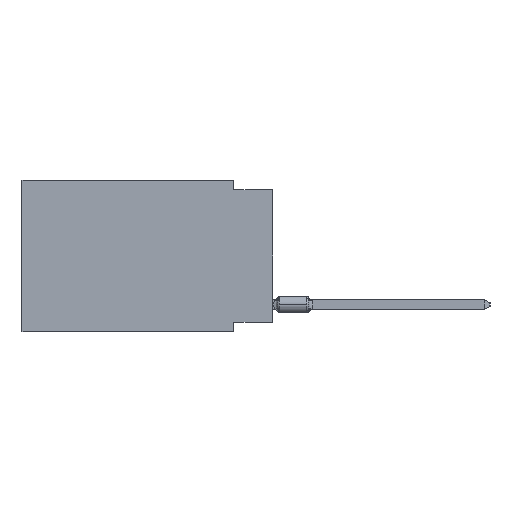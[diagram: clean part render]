
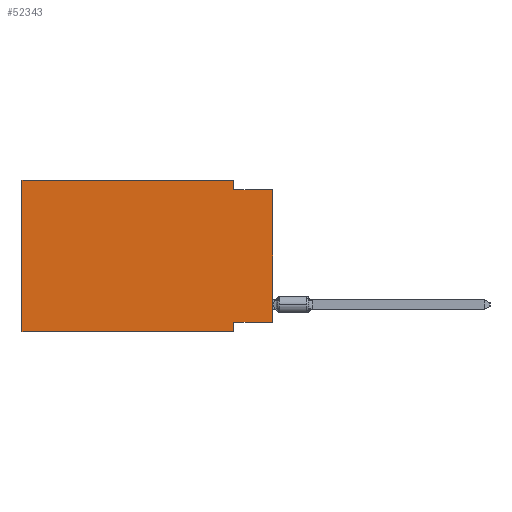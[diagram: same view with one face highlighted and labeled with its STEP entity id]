
A CAD part, left-side view. The second image highlights one B-rep face of the part: STEP entity #52343.
In plain terms, the highlighted planar face has unit normal (-1, 0, 0).
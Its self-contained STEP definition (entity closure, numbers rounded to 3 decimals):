
#439 = ORIENTED_EDGE ( 'NONE', *, *, #15975, .F. ) ;
#594 = DIRECTION ( 'NONE',  ( 0., -1., 0. ) ) ;
#1519 = DIRECTION ( 'NONE',  ( 1., 0., 0. ) ) ;
#2572 = EDGE_CURVE ( 'NONE', #44456, #15717, #60464, .T. ) ;
#2872 = DIRECTION ( 'NONE',  ( 0., 0., 1. ) ) ;
#3669 = CARTESIAN_POINT ( 'NONE',  ( 0., 16.383, 0. ) ) ;
#4310 = ORIENTED_EDGE ( 'NONE', *, *, #54827, .F. ) ;
#5152 = EDGE_CURVE ( 'NONE', #33757, #67316, #58648, .T. ) ;
#8845 = DIRECTION ( 'NONE',  ( 0., -1., 0. ) ) ;
#10815 = VECTOR ( 'NONE', #2872, 1000. ) ;
#11111 = CARTESIAN_POINT ( 'NONE',  ( 0., 2.54, -9.906 ) ) ;
#11464 = CARTESIAN_POINT ( 'NONE',  ( 0., 2.54, 0. ) ) ;
#12512 = VECTOR ( 'NONE', #8845, 1000. ) ;
#12862 = CARTESIAN_POINT ( 'NONE',  ( 0., 16.383, 0. ) ) ;
#13574 = DIRECTION ( 'NONE',  ( 0., -1., 0. ) ) ;
#13678 = LINE ( 'NONE', #3669, #12512 ) ;
#14468 = CARTESIAN_POINT ( 'NONE',  ( 0., 0., 0. ) ) ;
#15052 = CARTESIAN_POINT ( 'NONE',  ( 0., 2.54, -9.906 ) ) ;
#15717 = VERTEX_POINT ( 'NONE', #11111 ) ;
#15845 = CARTESIAN_POINT ( 'NONE',  ( 0., 0., -9.271 ) ) ;
#15975 = EDGE_CURVE ( 'NONE', #67316, #20374, #13678, .T. ) ;
#16639 = EDGE_CURVE ( 'NONE', #33757, #15717, #19100, .T. ) ;
#17919 = VECTOR ( 'NONE', #594, 1000. ) ;
#18137 = PLANE ( 'NONE',  #50820 ) ;
#19100 = LINE ( 'NONE', #41634, #67995 ) ;
#19553 = CARTESIAN_POINT ( 'NONE',  ( 0., 0., -0.635 ) ) ;
#19812 = DIRECTION ( 'NONE',  ( 0., 1., 0. ) ) ;
#20374 = VERTEX_POINT ( 'NONE', #34454 ) ;
#20508 = VERTEX_POINT ( 'NONE', #42528 ) ;
#24146 = ORIENTED_EDGE ( 'NONE', *, *, #67704, .F. ) ;
#27179 = LINE ( 'NONE', #29018, #17919 ) ;
#29018 = CARTESIAN_POINT ( 'NONE',  ( 0., 0., -0.635 ) ) ;
#30363 = VERTEX_POINT ( 'NONE', #19553 ) ;
#31337 = EDGE_CURVE ( 'NONE', #20374, #20508, #46146, .T. ) ;
#32254 = VECTOR ( 'NONE', #19812, 1000. ) ;
#33107 = DIRECTION ( 'NONE',  ( 0., 0., -1. ) ) ;
#33757 = VERTEX_POINT ( 'NONE', #69643 ) ;
#34454 = CARTESIAN_POINT ( 'NONE',  ( 0., 2.54, 0. ) ) ;
#36993 = DIRECTION ( 'NONE',  ( 0., 0., 1. ) ) ;
#38234 = ORIENTED_EDGE ( 'NONE', *, *, #31337, .F. ) ;
#41272 = LINE ( 'NONE', #52713, #32254 ) ;
#41634 = CARTESIAN_POINT ( 'NONE',  ( 0., 16.383, -9.906 ) ) ;
#42528 = CARTESIAN_POINT ( 'NONE',  ( 0., 2.54, -0.635 ) ) ;
#43493 = VECTOR ( 'NONE', #33107, 1000. ) ;
#44456 = VERTEX_POINT ( 'NONE', #46496 ) ;
#44555 = EDGE_LOOP ( 'NONE', ( #44778, #24146, #38234, #439, #54751, #67600, #47407, #4310 ) ) ;
#44778 = ORIENTED_EDGE ( 'NONE', *, *, #63929, .T. ) ;
#45044 = DIRECTION ( 'NONE',  ( 0., 0., -1. ) ) ;
#45253 = VECTOR ( 'NONE', #45044, 1000. ) ;
#45731 = CARTESIAN_POINT ( 'NONE',  ( 0., 16.383, 0. ) ) ;
#46146 = LINE ( 'NONE', #11464, #45253 ) ;
#46496 = CARTESIAN_POINT ( 'NONE',  ( 0., 2.54, -9.271 ) ) ;
#47407 = ORIENTED_EDGE ( 'NONE', *, *, #2572, .F. ) ;
#50820 = AXIS2_PLACEMENT_3D ( 'NONE', #52463, #1519, #64654 ) ;
#52343 = ADVANCED_FACE ( 'NONE', ( #58737 ), #18137, .F. ) ;
#52463 = CARTESIAN_POINT ( 'NONE',  ( 0., 16.383, 0. ) ) ;
#52713 = CARTESIAN_POINT ( 'NONE',  ( 0., 0., -9.271 ) ) ;
#54188 = VECTOR ( 'NONE', #36993, 1000. ) ;
#54751 = ORIENTED_EDGE ( 'NONE', *, *, #5152, .F. ) ;
#54827 = EDGE_CURVE ( 'NONE', #70318, #44456, #41272, .T. ) ;
#58648 = LINE ( 'NONE', #12862, #10815 ) ;
#58737 = FACE_OUTER_BOUND ( 'NONE', #44555, .T. ) ;
#59149 = LINE ( 'NONE', #14468, #54188 ) ;
#60464 = LINE ( 'NONE', #15052, #43493 ) ;
#63929 = EDGE_CURVE ( 'NONE', #70318, #30363, #59149, .T. ) ;
#64654 = DIRECTION ( 'NONE',  ( 0., 0., -1. ) ) ;
#67316 = VERTEX_POINT ( 'NONE', #45731 ) ;
#67600 = ORIENTED_EDGE ( 'NONE', *, *, #16639, .T. ) ;
#67704 = EDGE_CURVE ( 'NONE', #20508, #30363, #27179, .T. ) ;
#67995 = VECTOR ( 'NONE', #13574, 1000. ) ;
#69643 = CARTESIAN_POINT ( 'NONE',  ( 0., 16.383, -9.906 ) ) ;
#70318 = VERTEX_POINT ( 'NONE', #15845 ) ;
